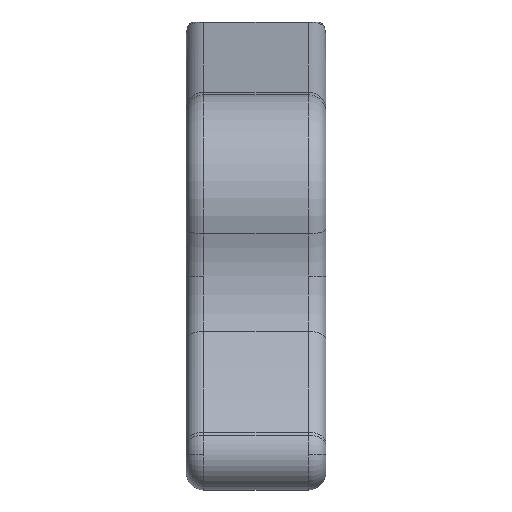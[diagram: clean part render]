
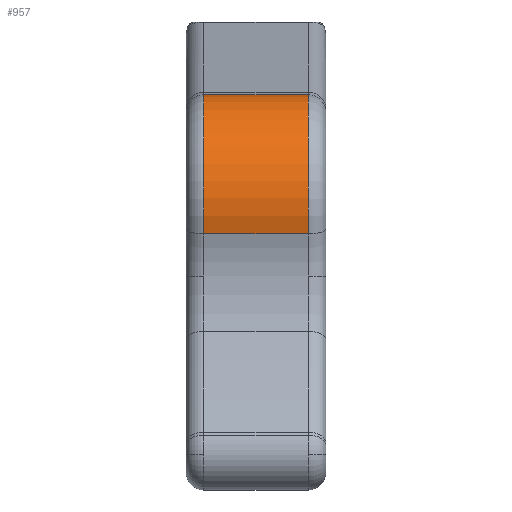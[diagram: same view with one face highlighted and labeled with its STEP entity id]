
A CAD part, top view. The second image highlights one B-rep face of the part: STEP entity #957.
In plain terms, the highlighted cylindrical face has radius 7.602 mm (diameter 15.203 mm), a partial arc.
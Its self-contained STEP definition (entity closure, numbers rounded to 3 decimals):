
#16 = DIRECTION ( 'NONE',  ( 1., 0., 0. ) ) ;
#47 = CARTESIAN_POINT ( 'NONE',  ( -26.45, -2.27, 7.255 ) ) ;
#117 = CIRCLE ( 'NONE', #1907, 7.602 ) ;
#159 = ORIENTED_EDGE ( 'NONE', *, *, #1519, .T. ) ;
#203 = VERTEX_POINT ( 'NONE', #388 ) ;
#248 = AXIS2_PLACEMENT_3D ( 'NONE', #558, #1663, #830 ) ;
#272 = CIRCLE ( 'NONE', #248, 7.602 ) ;
#368 = ORIENTED_EDGE ( 'NONE', *, *, #670, .T. ) ;
#388 = CARTESIAN_POINT ( 'NONE',  ( 3.699, -2.27, 7.255 ) ) ;
#448 = VERTEX_POINT ( 'NONE', #591 ) ;
#543 = CARTESIAN_POINT ( 'NONE',  ( -26.45, 7.535, -1.005 ) ) ;
#558 = CARTESIAN_POINT ( 'NONE',  ( 3.699, 0., 0. ) ) ;
#591 = CARTESIAN_POINT ( 'NONE',  ( 3.699, 7.535, -1.005 ) ) ;
#670 = EDGE_CURVE ( 'NONE', #1078, #203, #2003, .T. ) ;
#830 = DIRECTION ( 'NONE',  ( 0., 0., -1. ) ) ;
#871 = CARTESIAN_POINT ( 'NONE',  ( -3.699, -2.27, 7.255 ) ) ;
#895 = VECTOR ( 'NONE', #1154, 1000. ) ;
#912 = CARTESIAN_POINT ( 'NONE',  ( -3.699, 0., 0. ) ) ;
#938 = AXIS2_PLACEMENT_3D ( 'NONE', #1513, #1344, #2020 ) ;
#957 = ADVANCED_FACE ( 'NONE', ( #1573 ), #1971, .T. ) ;
#1070 = DIRECTION ( 'NONE',  ( 0., 0., -1. ) ) ;
#1078 = VERTEX_POINT ( 'NONE', #871 ) ;
#1116 = VECTOR ( 'NONE', #1783, 1000. ) ;
#1123 = EDGE_CURVE ( 'NONE', #448, #1768, #1763, .T. ) ;
#1154 = DIRECTION ( 'NONE',  ( -1., 0., 0. ) ) ;
#1344 = DIRECTION ( 'NONE',  ( 1., 0., 0. ) ) ;
#1355 = ORIENTED_EDGE ( 'NONE', *, *, #1123, .T. ) ;
#1367 = ORIENTED_EDGE ( 'NONE', *, *, #1905, .T. ) ;
#1513 = CARTESIAN_POINT ( 'NONE',  ( -26.45, 0., 0. ) ) ;
#1519 = EDGE_CURVE ( 'NONE', #203, #448, #272, .T. ) ;
#1573 = FACE_OUTER_BOUND ( 'NONE', #1937, .T. ) ;
#1663 = DIRECTION ( 'NONE',  ( -1., 0., 0. ) ) ;
#1763 = LINE ( 'NONE', #543, #895 ) ;
#1768 = VERTEX_POINT ( 'NONE', #1871 ) ;
#1783 = DIRECTION ( 'NONE',  ( 1., 0., 0. ) ) ;
#1871 = CARTESIAN_POINT ( 'NONE',  ( -3.699, 7.535, -1.005 ) ) ;
#1905 = EDGE_CURVE ( 'NONE', #1768, #1078, #117, .T. ) ;
#1907 = AXIS2_PLACEMENT_3D ( 'NONE', #912, #16, #1070 ) ;
#1937 = EDGE_LOOP ( 'NONE', ( #1355, #1367, #368, #159 ) ) ;
#1971 = CYLINDRICAL_SURFACE ( 'NONE', #938, 7.602 ) ;
#2003 = LINE ( 'NONE', #47, #1116 ) ;
#2020 = DIRECTION ( 'NONE',  ( 0., 0., -1. ) ) ;
